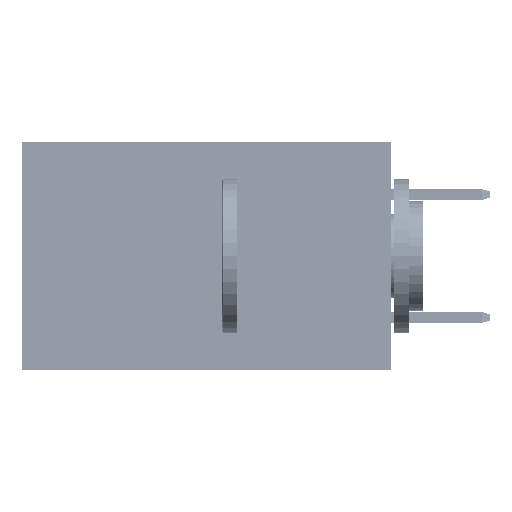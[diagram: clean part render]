
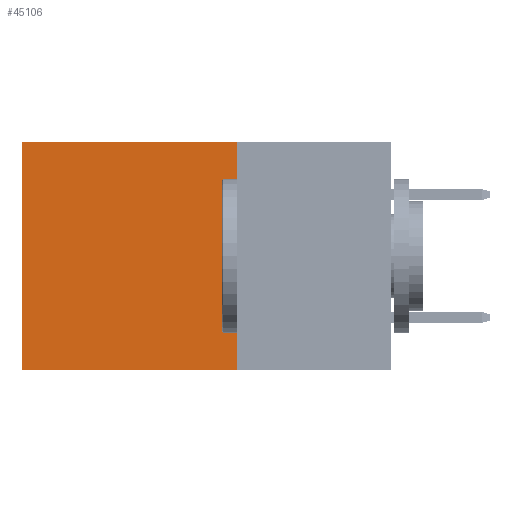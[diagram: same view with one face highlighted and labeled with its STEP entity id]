
A CAD part, left-side view. The second image highlights one B-rep face of the part: STEP entity #45106.
In plain terms, the highlighted planar face has unit normal (-1, 0, 0).
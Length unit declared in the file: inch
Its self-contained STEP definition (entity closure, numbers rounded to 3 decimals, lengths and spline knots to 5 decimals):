
#1054 = EDGE_CURVE ( 'NONE', #33281, #16674, #46418, .T. ) ;
#1226 = CARTESIAN_POINT ( 'NONE',  ( 0.2875, 0.25, 0. ) ) ;
#1498 = CARTESIAN_POINT ( 'NONE',  ( 0.2875, 0.25, 0. ) ) ;
#3662 = VERTEX_POINT ( 'NONE', #50881 ) ;
#5035 = VECTOR ( 'NONE', #6640, 39.37008 ) ;
#5481 = DIRECTION ( 'NONE',  ( 0., 0., -1. ) ) ;
#5851 = ORIENTED_EDGE ( 'NONE', *, *, #38215, .T. ) ;
#6228 = FACE_OUTER_BOUND ( 'NONE', #11945, .T. ) ;
#6640 = DIRECTION ( 'NONE',  ( 0., 0., -1. ) ) ;
#7541 = DIRECTION ( 'NONE',  ( 0., 0., -1. ) ) ;
#7601 = VECTOR ( 'NONE', #48711, 39.37008 ) ;
#11945 = EDGE_LOOP ( 'NONE', ( #5851, #23017, #31706, #40090 ) ) ;
#12137 = VECTOR ( 'NONE', #7541, 39.37008 ) ;
#13360 = LINE ( 'NONE', #19350, #12137 ) ;
#15611 = LINE ( 'NONE', #34298, #5035 ) ;
#16674 = VERTEX_POINT ( 'NONE', #20068 ) ;
#18738 = CARTESIAN_POINT ( 'NONE',  ( 0.2875, 0.25, 0. ) ) ;
#19350 = CARTESIAN_POINT ( 'NONE',  ( 0.2875, 0.6, 0. ) ) ;
#20068 = CARTESIAN_POINT ( 'NONE',  ( 0.2875, 0.6, -0.37 ) ) ;
#23017 = ORIENTED_EDGE ( 'NONE', *, *, #1054, .F. ) ;
#24145 = VECTOR ( 'NONE', #42422, 39.37008 ) ;
#24446 = AXIS2_PLACEMENT_3D ( 'NONE', #1498, #29306, #5481 ) ;
#27180 = EDGE_CURVE ( 'NONE', #29807, #3662, #39294, .T. ) ;
#29306 = DIRECTION ( 'NONE',  ( 1., 0., 0. ) ) ;
#29807 = VERTEX_POINT ( 'NONE', #18738 ) ;
#31706 = ORIENTED_EDGE ( 'NONE', *, *, #41141, .F. ) ;
#33139 = PLANE ( 'NONE',  #24446 ) ;
#33281 = VERTEX_POINT ( 'NONE', #33664 ) ;
#33664 = CARTESIAN_POINT ( 'NONE',  ( 0.2875, 0.25, -0.37 ) ) ;
#34298 = CARTESIAN_POINT ( 'NONE',  ( 0.2875, 0.25, 0. ) ) ;
#38215 = EDGE_CURVE ( 'NONE', #3662, #16674, #13360, .T. ) ;
#39294 = LINE ( 'NONE', #1226, #7601 ) ;
#40090 = ORIENTED_EDGE ( 'NONE', *, *, #27180, .T. ) ;
#41141 = EDGE_CURVE ( 'NONE', #29807, #33281, #15611, .T. ) ;
#42422 = DIRECTION ( 'NONE',  ( 0., 1., 0. ) ) ;
#45106 = ADVANCED_FACE ( 'NONE', ( #6228 ), #33139, .F. ) ;
#46393 = CARTESIAN_POINT ( 'NONE',  ( 0.2875, 0.25, -0.37 ) ) ;
#46418 = LINE ( 'NONE', #46393, #24145 ) ;
#48711 = DIRECTION ( 'NONE',  ( 0., 1., 0. ) ) ;
#50881 = CARTESIAN_POINT ( 'NONE',  ( 0.2875, 0.6, 0. ) ) ;
